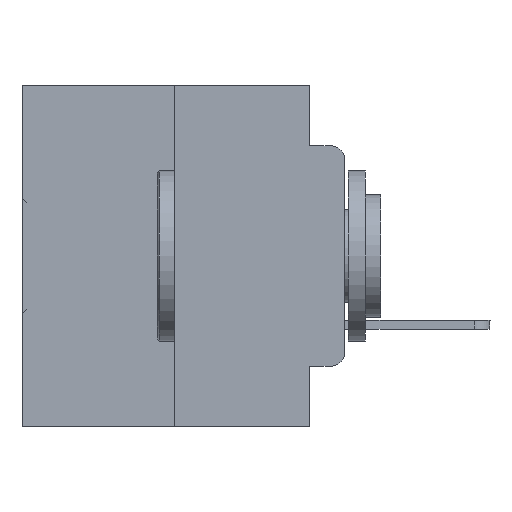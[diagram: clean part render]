
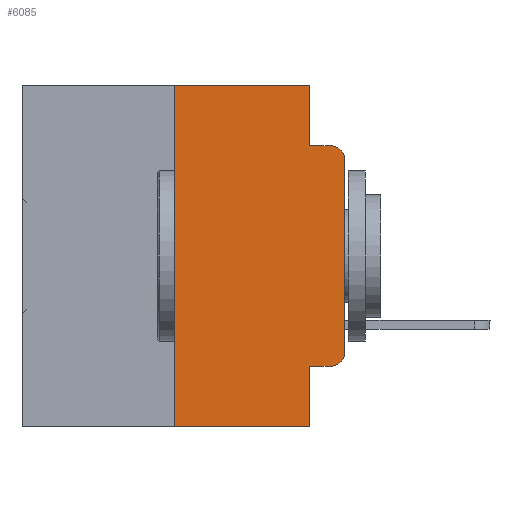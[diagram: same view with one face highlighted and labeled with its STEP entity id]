
A CAD part, left-side view. The second image highlights one B-rep face of the part: STEP entity #6085.
In plain terms, the highlighted planar face has unit normal (-1, 0, 0).
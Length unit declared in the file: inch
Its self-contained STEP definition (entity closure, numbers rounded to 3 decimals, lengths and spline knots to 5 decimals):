
#816 = EDGE_CURVE ( 'NONE', #29441, #1321, #34102, .T. ) ;
#834 = CARTESIAN_POINT ( 'NONE',  ( 0., 0.473, 0. ) ) ;
#1321 = VERTEX_POINT ( 'NONE', #28110 ) ;
#1753 = LINE ( 'NONE', #12719, #17335 ) ;
#1956 = LINE ( 'NONE', #30370, #34366 ) ;
#2091 = DIRECTION ( 'NONE',  ( 0., 0., -1. ) ) ;
#2504 = CARTESIAN_POINT ( 'NONE',  ( 0., 0.051, 0. ) ) ;
#3110 = ORIENTED_EDGE ( 'NONE', *, *, #21425, .T. ) ;
#3235 = EDGE_CURVE ( 'NONE', #21815, #28755, #31931, .T. ) ;
#3433 = CIRCLE ( 'NONE', #8399, 0.02 ) ;
#3674 = EDGE_CURVE ( 'NONE', #30475, #15357, #8261, .T. ) ;
#3729 = EDGE_CURVE ( 'NONE', #17197, #28755, #17580, .T. ) ;
#4006 = CARTESIAN_POINT ( 'NONE',  ( 0., 0.473, 0. ) ) ;
#4216 = ORIENTED_EDGE ( 'NONE', *, *, #28653, .T. ) ;
#4274 = ORIENTED_EDGE ( 'NONE', *, *, #20070, .F. ) ;
#4480 = CARTESIAN_POINT ( 'NONE',  ( 0., 0.051, 0. ) ) ;
#4544 = CARTESIAN_POINT ( 'NONE',  ( 0., 0.02, -0.0885 ) ) ;
#5337 = ORIENTED_EDGE ( 'NONE', *, *, #34369, .F. ) ;
#5608 = DIRECTION ( 'NONE',  ( 0., -1., 0. ) ) ;
#6085 = ADVANCED_FACE ( 'NONE', ( #33441 ), #17603, .F. ) ;
#6545 = VECTOR ( 'NONE', #16228, 39.37008 ) ;
#8261 = LINE ( 'NONE', #10840, #30137 ) ;
#8399 = AXIS2_PLACEMENT_3D ( 'NONE', #19782, #33349, #25648 ) ;
#8713 = EDGE_CURVE ( 'NONE', #16819, #30475, #14773, .T. ) ;
#10559 = AXIS2_PLACEMENT_3D ( 'NONE', #4006, #14759, #25575 ) ;
#10840 = CARTESIAN_POINT ( 'NONE',  ( 0., 0.051, 0. ) ) ;
#11738 = VECTOR ( 'NONE', #5608, 39.37008 ) ;
#11741 = DIRECTION ( 'NONE',  ( 0., -1., 0. ) ) ;
#12719 = CARTESIAN_POINT ( 'NONE',  ( 0., 0.25, 0. ) ) ;
#12780 = CARTESIAN_POINT ( 'NONE',  ( 0., 0.25, 0. ) ) ;
#13441 = EDGE_CURVE ( 'NONE', #18932, #20948, #3433, .T. ) ;
#14414 = DIRECTION ( 'NONE',  ( 0., -1., 0. ) ) ;
#14759 = DIRECTION ( 'NONE',  ( 1., 0., 0. ) ) ;
#14773 = LINE ( 'NONE', #834, #21544 ) ;
#15357 = VERTEX_POINT ( 'NONE', #17997 ) ;
#15603 = LINE ( 'NONE', #21774, #11738 ) ;
#15813 = CARTESIAN_POINT ( 'NONE',  ( 0., 0.02, -0.3915 ) ) ;
#16228 = DIRECTION ( 'NONE',  ( 0., 0., -1. ) ) ;
#16819 = VERTEX_POINT ( 'NONE', #12780 ) ;
#17197 = VERTEX_POINT ( 'NONE', #19999 ) ;
#17335 = VECTOR ( 'NONE', #28613, 39.37008 ) ;
#17580 = LINE ( 'NONE', #2504, #6545 ) ;
#17603 = PLANE ( 'NONE',  #10559 ) ;
#17648 = VECTOR ( 'NONE', #11741, 39.37008 ) ;
#17672 = ORIENTED_EDGE ( 'NONE', *, *, #8713, .F. ) ;
#17701 = AXIS2_PLACEMENT_3D ( 'NONE', #15813, #26146, #2091 ) ;
#17997 = CARTESIAN_POINT ( 'NONE',  ( 0., 0.051, -0.0885 ) ) ;
#18932 = VERTEX_POINT ( 'NONE', #20437 ) ;
#19040 = DIRECTION ( 'NONE',  ( 0., 0., -1. ) ) ;
#19782 = CARTESIAN_POINT ( 'NONE',  ( 0., 0.02, -0.1085 ) ) ;
#19999 = CARTESIAN_POINT ( 'NONE',  ( 0., 0.051, -0.4115 ) ) ;
#20070 = EDGE_CURVE ( 'NONE', #15357, #20948, #15603, .T. ) ;
#20140 = DIRECTION ( 'NONE',  ( 0., -1., 0. ) ) ;
#20437 = CARTESIAN_POINT ( 'NONE',  ( 0., 0., -0.1085 ) ) ;
#20567 = DIRECTION ( 'NONE',  ( 0., 0., 1. ) ) ;
#20948 = VERTEX_POINT ( 'NONE', #4544 ) ;
#21425 = EDGE_CURVE ( 'NONE', #1321, #18932, #1956, .T. ) ;
#21544 = VECTOR ( 'NONE', #14414, 39.37008 ) ;
#21774 = CARTESIAN_POINT ( 'NONE',  ( 0., 0.051, -0.0885 ) ) ;
#21815 = VERTEX_POINT ( 'NONE', #22235 ) ;
#22207 = ORIENTED_EDGE ( 'NONE', *, *, #816, .T. ) ;
#22235 = CARTESIAN_POINT ( 'NONE',  ( 0., 0.25, -0.5 ) ) ;
#23576 = ORIENTED_EDGE ( 'NONE', *, *, #3235, .T. ) ;
#24579 = CARTESIAN_POINT ( 'NONE',  ( 0., 0.02, -0.4115 ) ) ;
#25575 = DIRECTION ( 'NONE',  ( 0., 0., -1. ) ) ;
#25648 = DIRECTION ( 'NONE',  ( 0., 0., -1. ) ) ;
#26146 = DIRECTION ( 'NONE',  ( -1., 0., 0. ) ) ;
#28110 = CARTESIAN_POINT ( 'NONE',  ( 0., 0., -0.3915 ) ) ;
#28613 = DIRECTION ( 'NONE',  ( 0., 0., 1. ) ) ;
#28653 = EDGE_CURVE ( 'NONE', #17197, #29441, #29039, .T. ) ;
#28755 = VERTEX_POINT ( 'NONE', #29468 ) ;
#29039 = LINE ( 'NONE', #30668, #34459 ) ;
#29441 = VERTEX_POINT ( 'NONE', #24579 ) ;
#29468 = CARTESIAN_POINT ( 'NONE',  ( 0., 0.051, -0.5 ) ) ;
#29944 = ORIENTED_EDGE ( 'NONE', *, *, #3729, .F. ) ;
#30137 = VECTOR ( 'NONE', #19040, 39.37008 ) ;
#30370 = CARTESIAN_POINT ( 'NONE',  ( 0., 0., 0. ) ) ;
#30475 = VERTEX_POINT ( 'NONE', #4480 ) ;
#30668 = CARTESIAN_POINT ( 'NONE',  ( 0., 0.051, -0.4115 ) ) ;
#31931 = LINE ( 'NONE', #33005, #17648 ) ;
#32895 = ORIENTED_EDGE ( 'NONE', *, *, #3674, .F. ) ;
#33005 = CARTESIAN_POINT ( 'NONE',  ( 0., 0.473, -0.5 ) ) ;
#33349 = DIRECTION ( 'NONE',  ( -1., 0., 0. ) ) ;
#33441 = FACE_OUTER_BOUND ( 'NONE', #34112, .T. ) ;
#34102 = CIRCLE ( 'NONE', #17701, 0.02 ) ;
#34112 = EDGE_LOOP ( 'NONE', ( #3110, #34507, #4274, #32895, #17672, #5337, #23576, #29944, #4216, #22207 ) ) ;
#34366 = VECTOR ( 'NONE', #20567, 39.37008 ) ;
#34369 = EDGE_CURVE ( 'NONE', #21815, #16819, #1753, .T. ) ;
#34459 = VECTOR ( 'NONE', #20140, 39.37008 ) ;
#34507 = ORIENTED_EDGE ( 'NONE', *, *, #13441, .T. ) ;
